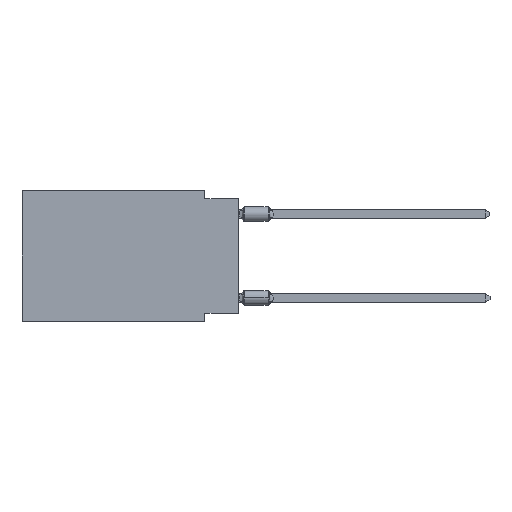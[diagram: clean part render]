
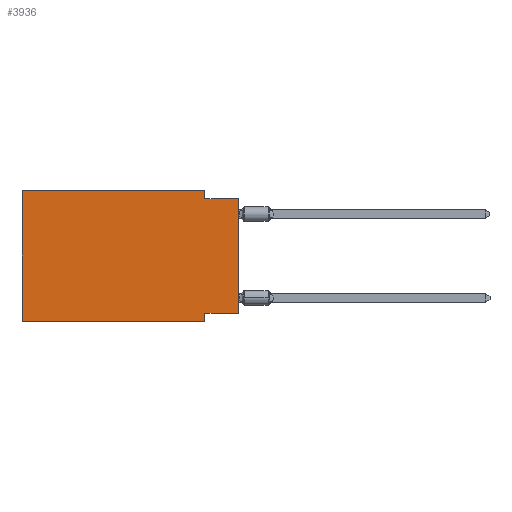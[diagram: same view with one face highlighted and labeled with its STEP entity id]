
A CAD part, left-side view. The second image highlights one B-rep face of the part: STEP entity #3936.
In plain terms, the highlighted planar face has unit normal (-1, 0, 0).
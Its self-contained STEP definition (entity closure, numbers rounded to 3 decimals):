
#728 = CARTESIAN_POINT ( 'NONE',  ( 0., 2.54, -9.906 ) ) ;
#791 = CARTESIAN_POINT ( 'NONE',  ( 0., 0., -9.271 ) ) ;
#996 = CARTESIAN_POINT ( 'NONE',  ( 0., 2.54, 0. ) ) ;
#1027 = CARTESIAN_POINT ( 'NONE',  ( 0., 0., 0. ) ) ;
#1037 = VERTEX_POINT ( 'NONE', #12613 ) ;
#1227 = EDGE_CURVE ( 'NONE', #6888, #6146, #7012, .T. ) ;
#1484 = CARTESIAN_POINT ( 'NONE',  ( 0., 16.383, 0. ) ) ;
#1682 = CARTESIAN_POINT ( 'NONE',  ( 0., 16.383, -9.906 ) ) ;
#1810 = VERTEX_POINT ( 'NONE', #4192 ) ;
#1942 = DIRECTION ( 'NONE',  ( 0., 0., -1. ) ) ;
#2126 = VECTOR ( 'NONE', #9738, 1000. ) ;
#2419 = EDGE_CURVE ( 'NONE', #1810, #1037, #4497, .T. ) ;
#2608 = VERTEX_POINT ( 'NONE', #4079 ) ;
#2880 = DIRECTION ( 'NONE',  ( 0., 0., -1. ) ) ;
#2911 = CARTESIAN_POINT ( 'NONE',  ( 0., 16.383, 0. ) ) ;
#2965 = EDGE_CURVE ( 'NONE', #1810, #2608, #5186, .T. ) ;
#3308 = EDGE_CURVE ( 'NONE', #8277, #6146, #4661, .T. ) ;
#3617 = CARTESIAN_POINT ( 'NONE',  ( 0., 2.54, -9.271 ) ) ;
#3640 = ORIENTED_EDGE ( 'NONE', *, *, #8883, .F. ) ;
#3907 = FACE_OUTER_BOUND ( 'NONE', #9054, .T. ) ;
#3936 = ADVANCED_FACE ( 'NONE', ( #3907 ), #7935, .F. ) ;
#4079 = CARTESIAN_POINT ( 'NONE',  ( 0., 16.383, 0. ) ) ;
#4192 = CARTESIAN_POINT ( 'NONE',  ( 0., 16.383, -9.906 ) ) ;
#4391 = ORIENTED_EDGE ( 'NONE', *, *, #3308, .F. ) ;
#4489 = DIRECTION ( 'NONE',  ( 0., -1., 0. ) ) ;
#4497 = LINE ( 'NONE', #1682, #9879 ) ;
#4661 = LINE ( 'NONE', #11948, #6544 ) ;
#5186 = LINE ( 'NONE', #7175, #10941 ) ;
#5258 = ORIENTED_EDGE ( 'NONE', *, *, #6895, .F. ) ;
#5587 = ORIENTED_EDGE ( 'NONE', *, *, #2965, .F. ) ;
#5799 = ORIENTED_EDGE ( 'NONE', *, *, #12648, .F. ) ;
#5904 = VECTOR ( 'NONE', #2880, 1000. ) ;
#6146 = VERTEX_POINT ( 'NONE', #10928 ) ;
#6156 = DIRECTION ( 'NONE',  ( 0., 0., 1. ) ) ;
#6420 = ORIENTED_EDGE ( 'NONE', *, *, #2419, .T. ) ;
#6544 = VECTOR ( 'NONE', #12681, 1000. ) ;
#6885 = LINE ( 'NONE', #728, #8935 ) ;
#6888 = VERTEX_POINT ( 'NONE', #791 ) ;
#6891 = CARTESIAN_POINT ( 'NONE',  ( 0., 0., -9.271 ) ) ;
#6895 = EDGE_CURVE ( 'NONE', #10931, #1037, #6885, .T. ) ;
#6947 = DIRECTION ( 'NONE',  ( 1., 0., 0. ) ) ;
#7012 = LINE ( 'NONE', #1027, #7606 ) ;
#7175 = CARTESIAN_POINT ( 'NONE',  ( 0., 16.383, 0. ) ) ;
#7606 = VECTOR ( 'NONE', #6156, 1000. ) ;
#7753 = LINE ( 'NONE', #6891, #2126 ) ;
#7935 = PLANE ( 'NONE',  #8667 ) ;
#8028 = DIRECTION ( 'NONE',  ( 0., 0., 1. ) ) ;
#8277 = VERTEX_POINT ( 'NONE', #9128 ) ;
#8389 = LINE ( 'NONE', #1484, #10405 ) ;
#8667 = AXIS2_PLACEMENT_3D ( 'NONE', #2911, #6947, #1942 ) ;
#8883 = EDGE_CURVE ( 'NONE', #2608, #9680, #8389, .T. ) ;
#8935 = VECTOR ( 'NONE', #12920, 1000. ) ;
#9054 = EDGE_LOOP ( 'NONE', ( #9191, #4391, #11193, #3640, #5587, #6420, #5258, #5799 ) ) ;
#9128 = CARTESIAN_POINT ( 'NONE',  ( 0., 2.54, -0.635 ) ) ;
#9191 = ORIENTED_EDGE ( 'NONE', *, *, #1227, .T. ) ;
#9680 = VERTEX_POINT ( 'NONE', #9729 ) ;
#9729 = CARTESIAN_POINT ( 'NONE',  ( 0., 2.54, 0. ) ) ;
#9738 = DIRECTION ( 'NONE',  ( 0., 1., 0. ) ) ;
#9879 = VECTOR ( 'NONE', #11476, 1000. ) ;
#10405 = VECTOR ( 'NONE', #4489, 1000. ) ;
#10928 = CARTESIAN_POINT ( 'NONE',  ( 0., 0., -0.635 ) ) ;
#10931 = VERTEX_POINT ( 'NONE', #3617 ) ;
#10941 = VECTOR ( 'NONE', #8028, 1000. ) ;
#11193 = ORIENTED_EDGE ( 'NONE', *, *, #12247, .F. ) ;
#11476 = DIRECTION ( 'NONE',  ( 0., -1., 0. ) ) ;
#11842 = LINE ( 'NONE', #996, #5904 ) ;
#11948 = CARTESIAN_POINT ( 'NONE',  ( 0., 0., -0.635 ) ) ;
#12247 = EDGE_CURVE ( 'NONE', #9680, #8277, #11842, .T. ) ;
#12613 = CARTESIAN_POINT ( 'NONE',  ( 0., 2.54, -9.906 ) ) ;
#12648 = EDGE_CURVE ( 'NONE', #6888, #10931, #7753, .T. ) ;
#12681 = DIRECTION ( 'NONE',  ( 0., -1., 0. ) ) ;
#12920 = DIRECTION ( 'NONE',  ( 0., 0., -1. ) ) ;
